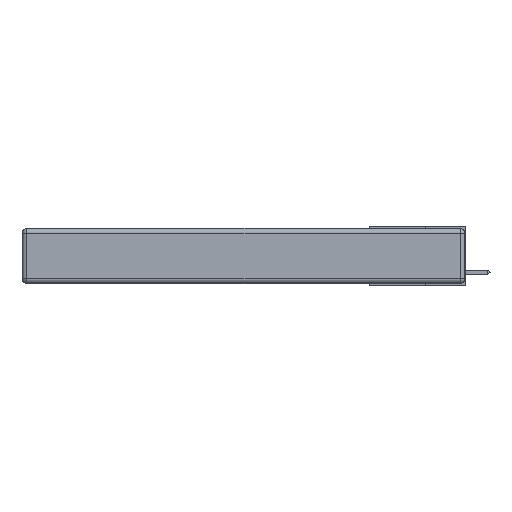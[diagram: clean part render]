
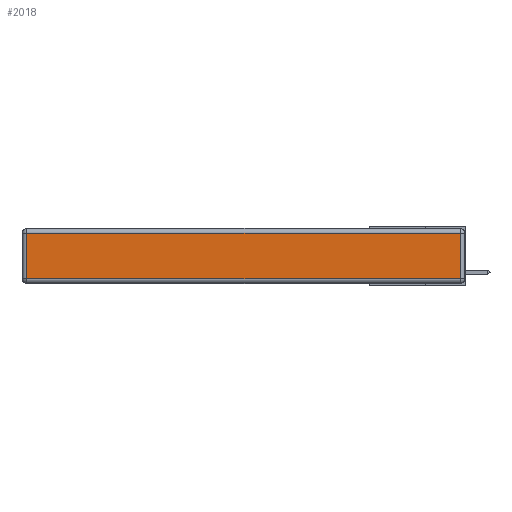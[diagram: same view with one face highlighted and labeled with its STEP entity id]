
A CAD part, left-side view. The second image highlights one B-rep face of the part: STEP entity #2018.
In plain terms, the highlighted planar face has unit normal (-1, 0, 0).
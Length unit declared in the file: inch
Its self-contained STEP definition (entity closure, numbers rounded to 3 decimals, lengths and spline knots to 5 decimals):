
#1057 = VERTEX_POINT ( 'NONE', #12194 ) ;
#1829 = AXIS2_PLACEMENT_3D ( 'NONE', #16691, #18146, #5123 ) ;
#2018 = ADVANCED_FACE ( 'NONE', ( #16640 ), #7992, .T. ) ;
#3142 = EDGE_LOOP ( 'NONE', ( #3469, #10972, #17652, #16651 ) ) ;
#3469 = ORIENTED_EDGE ( 'NONE', *, *, #6071, .T. ) ;
#3973 = DIRECTION ( 'NONE',  ( 0., -1., 0. ) ) ;
#4592 = CARTESIAN_POINT ( 'NONE',  ( 0., 2.72, -0.313 ) ) ;
#5011 = VECTOR ( 'NONE', #11097, 39.37008 ) ;
#5123 = DIRECTION ( 'NONE',  ( 0., 0., 1. ) ) ;
#6071 = EDGE_CURVE ( 'NONE', #10043, #15303, #18113, .T. ) ;
#6411 = VECTOR ( 'NONE', #15759, 39.37008 ) ;
#6999 = CARTESIAN_POINT ( 'NONE',  ( 0., 0.03, -0.313 ) ) ;
#7356 = VECTOR ( 'NONE', #9332, 39.37008 ) ;
#7418 = EDGE_CURVE ( 'NONE', #15303, #1057, #8915, .T. ) ;
#7992 = PLANE ( 'NONE',  #1829 ) ;
#8863 = EDGE_CURVE ( 'NONE', #9326, #10043, #12231, .T. ) ;
#8915 = LINE ( 'NONE', #16528, #7356 ) ;
#9045 = LINE ( 'NONE', #9232, #5011 ) ;
#9232 = CARTESIAN_POINT ( 'NONE',  ( 0., 2.75, -0.03 ) ) ;
#9326 = VERTEX_POINT ( 'NONE', #16122 ) ;
#9332 = DIRECTION ( 'NONE',  ( 0., 0., 1. ) ) ;
#10043 = VERTEX_POINT ( 'NONE', #4592 ) ;
#10262 = CARTESIAN_POINT ( 'NONE',  ( 0., 2.72, -0.343 ) ) ;
#10972 = ORIENTED_EDGE ( 'NONE', *, *, #7418, .T. ) ;
#11097 = DIRECTION ( 'NONE',  ( 0., 1., 0. ) ) ;
#12194 = CARTESIAN_POINT ( 'NONE',  ( 0., 0.03, -0.03 ) ) ;
#12231 = LINE ( 'NONE', #10262, #6411 ) ;
#12464 = EDGE_CURVE ( 'NONE', #1057, #9326, #9045, .T. ) ;
#13378 = VECTOR ( 'NONE', #3973, 39.37008 ) ;
#14122 = CARTESIAN_POINT ( 'NONE',  ( 0., 0., -0.313 ) ) ;
#15303 = VERTEX_POINT ( 'NONE', #6999 ) ;
#15759 = DIRECTION ( 'NONE',  ( 0., 0., -1. ) ) ;
#16122 = CARTESIAN_POINT ( 'NONE',  ( 0., 2.72, -0.03 ) ) ;
#16528 = CARTESIAN_POINT ( 'NONE',  ( 0., 0.03, -0.343 ) ) ;
#16640 = FACE_OUTER_BOUND ( 'NONE', #3142, .T. ) ;
#16651 = ORIENTED_EDGE ( 'NONE', *, *, #8863, .T. ) ;
#16691 = CARTESIAN_POINT ( 'NONE',  ( 0., 0., -0.343 ) ) ;
#17652 = ORIENTED_EDGE ( 'NONE', *, *, #12464, .T. ) ;
#18113 = LINE ( 'NONE', #14122, #13378 ) ;
#18146 = DIRECTION ( 'NONE',  ( -1., 0., 0. ) ) ;
